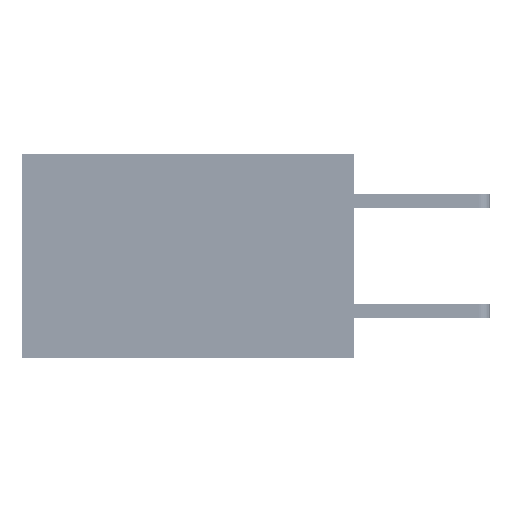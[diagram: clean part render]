
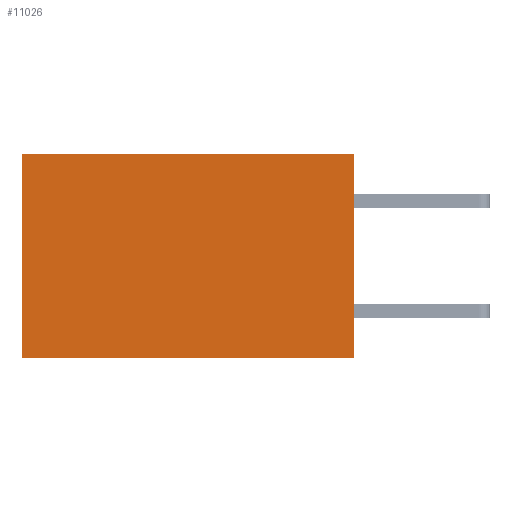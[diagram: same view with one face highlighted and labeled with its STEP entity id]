
A CAD part, left-side view. The second image highlights one B-rep face of the part: STEP entity #11026.
In plain terms, the highlighted planar face has unit normal (-1, 0, 0).
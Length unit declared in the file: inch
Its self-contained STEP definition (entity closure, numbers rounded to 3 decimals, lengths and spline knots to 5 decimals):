
#1664 = CARTESIAN_POINT ( 'NONE',  ( 0.2875, 0., -0.37 ) ) ;
#2836 = LINE ( 'NONE', #8679, #27048 ) ;
#6208 = LINE ( 'NONE', #1664, #13095 ) ;
#6437 = CARTESIAN_POINT ( 'NONE',  ( 0.2875, 0.6, 0. ) ) ;
#7358 = LINE ( 'NONE', #19249, #17483 ) ;
#8477 = VERTEX_POINT ( 'NONE', #21468 ) ;
#8679 = CARTESIAN_POINT ( 'NONE',  ( 0.2875, 0., 0. ) ) ;
#8916 = VECTOR ( 'NONE', #14032, 39.37008 ) ;
#9531 = CARTESIAN_POINT ( 'NONE',  ( 0.2875, 0., 0. ) ) ;
#10682 = DIRECTION ( 'NONE',  ( 0., 0., -1. ) ) ;
#11026 = ADVANCED_FACE ( 'NONE', ( #23520 ), #20320, .F. ) ;
#11959 = VERTEX_POINT ( 'NONE', #6437 ) ;
#12358 = EDGE_CURVE ( 'NONE', #13691, #11959, #2836, .T. ) ;
#12709 = DIRECTION ( 'NONE',  ( 0., 1., 0. ) ) ;
#12736 = EDGE_LOOP ( 'NONE', ( #21292, #37064, #30264, #33926 ) ) ;
#13095 = VECTOR ( 'NONE', #27569, 39.37008 ) ;
#13691 = VERTEX_POINT ( 'NONE', #9531 ) ;
#14032 = DIRECTION ( 'NONE',  ( 0., 0., -1. ) ) ;
#14909 = DIRECTION ( 'NONE',  ( 1., 0., 0. ) ) ;
#16688 = LINE ( 'NONE', #37520, #8916 ) ;
#17483 = VECTOR ( 'NONE', #10682, 39.37008 ) ;
#17655 = CARTESIAN_POINT ( 'NONE',  ( 0.2875, 0., 0. ) ) ;
#17807 = AXIS2_PLACEMENT_3D ( 'NONE', #17655, #14909, #26686 ) ;
#19249 = CARTESIAN_POINT ( 'NONE',  ( 0.2875, 0., 0. ) ) ;
#20320 = PLANE ( 'NONE',  #17807 ) ;
#20377 = EDGE_CURVE ( 'NONE', #13691, #8477, #7358, .T. ) ;
#21292 = ORIENTED_EDGE ( 'NONE', *, *, #21772, .T. ) ;
#21468 = CARTESIAN_POINT ( 'NONE',  ( 0.2875, 0., -0.37 ) ) ;
#21772 = EDGE_CURVE ( 'NONE', #11959, #23071, #16688, .T. ) ;
#23071 = VERTEX_POINT ( 'NONE', #23857 ) ;
#23520 = FACE_OUTER_BOUND ( 'NONE', #12736, .T. ) ;
#23857 = CARTESIAN_POINT ( 'NONE',  ( 0.2875, 0.6, -0.37 ) ) ;
#26014 = EDGE_CURVE ( 'NONE', #8477, #23071, #6208, .T. ) ;
#26686 = DIRECTION ( 'NONE',  ( 0., 0., -1. ) ) ;
#27048 = VECTOR ( 'NONE', #12709, 39.37008 ) ;
#27569 = DIRECTION ( 'NONE',  ( 0., 1., 0. ) ) ;
#30264 = ORIENTED_EDGE ( 'NONE', *, *, #20377, .F. ) ;
#33926 = ORIENTED_EDGE ( 'NONE', *, *, #12358, .T. ) ;
#37064 = ORIENTED_EDGE ( 'NONE', *, *, #26014, .F. ) ;
#37520 = CARTESIAN_POINT ( 'NONE',  ( 0.2875, 0.6, 0. ) ) ;
